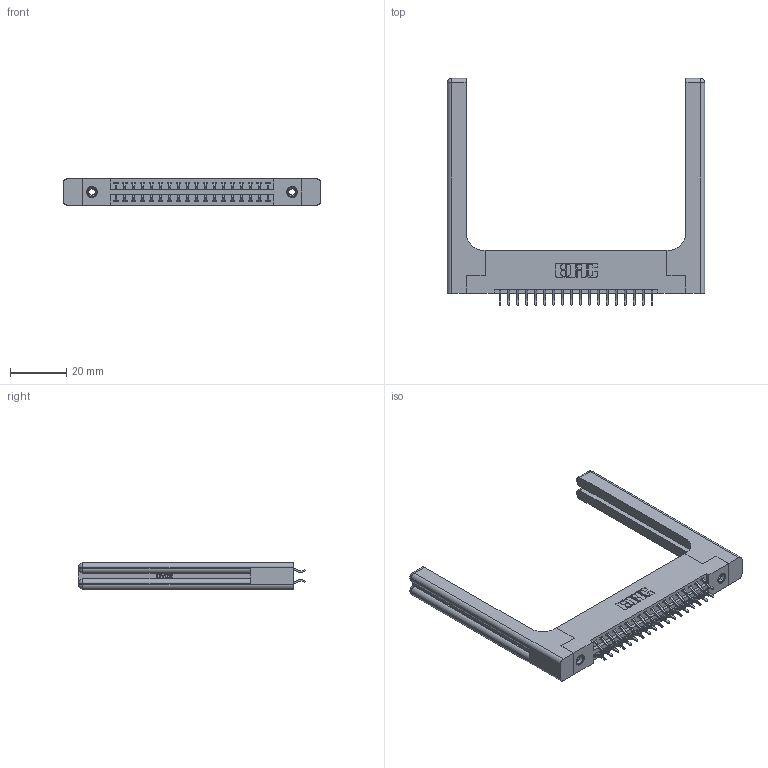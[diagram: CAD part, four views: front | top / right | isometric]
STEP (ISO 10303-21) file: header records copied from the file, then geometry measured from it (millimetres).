
FILE_DESCRIPTION (( 'STEP AP203' ), '1' );
FILE_NAME ('346-036-556-258.STEP', '2022-05-19T22:08:55', ( '' ), ( '' ), 'SwSTEP 2.0', 'SolidWorks 2020', '' );
FILE_SCHEMA (( 'CONFIG_CONTROL_DESIGN' ));
Length unit declared in the file: inch
Products named in the file (5): 345-292-001_556 Tail; 346-036-556-258; 346-220-058_345-220-058; 346 Part_Flush Mounting Lugs - 0.156 Dia-TH; 345-250-001_345-250-001-102
Assembly tree (41 placements, depth 2):
  346-036-556-258
    346 Part_Flush Mounting Lugs - 0.156 Dia-TH
    345-292-001_556 Tail  x36
    345-250-001_345-250-001-102  x2
    346-220-058_345-220-058  x2
Bounding box: 91.21 x 80.53 x 9.4 mm (x, y, z)
Volume: 16182.6 mm3; surface area: 16539.3 mm2
Topology: 41 solids, 41 shells, 2480 faces, 7259 edges, 4770 vertices
Faces by surface type: plane 1642, cylinder 778, bspline 36, cone 12, sphere 8, torus 4
Entity records: 20796 total; most frequent: CARTESIAN_POINT 4487, ORIENTED_EDGE 3204, DIRECTION 2926, EDGE_CURVE 1602, VECTOR 1298, LINE 1298, VERTEX_POINT 1058, AXIS2_PLACEMENT_3D 814
